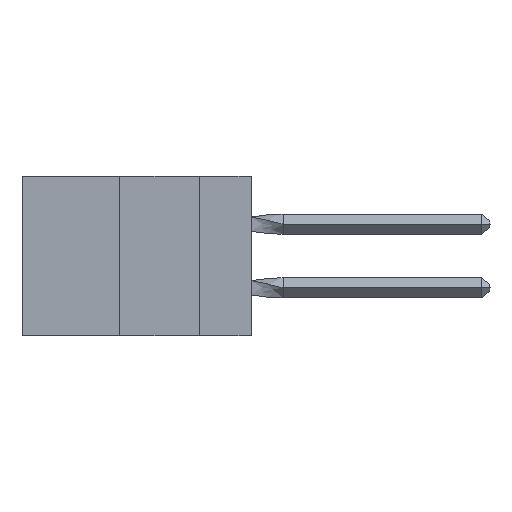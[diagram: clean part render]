
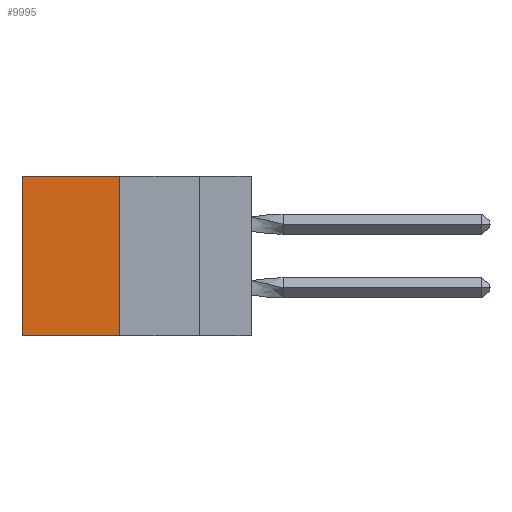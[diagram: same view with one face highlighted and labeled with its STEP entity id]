
A CAD part, left-side view. The second image highlights one B-rep face of the part: STEP entity #9995.
In plain terms, the highlighted planar face has unit normal (-1, 0, 0).
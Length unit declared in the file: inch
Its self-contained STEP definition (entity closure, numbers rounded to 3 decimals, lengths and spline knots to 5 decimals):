
#603 = LINE ( 'NONE', #24592, #18379 ) ;
#637 = CARTESIAN_POINT ( 'NONE',  ( 0.305, 0.413, 0. ) ) ;
#692 = FACE_OUTER_BOUND ( 'NONE', #27209, .T. ) ;
#999 = LINE ( 'NONE', #6734, #24939 ) ;
#2280 = DIRECTION ( 'NONE',  ( 0., 0., -1. ) ) ;
#2689 = VERTEX_POINT ( 'NONE', #19677 ) ;
#2735 = VECTOR ( 'NONE', #25598, 39.37008 ) ;
#3597 = PLANE ( 'NONE',  #12954 ) ;
#4885 = VERTEX_POINT ( 'NONE', #9033 ) ;
#5884 = EDGE_CURVE ( 'NONE', #26504, #4885, #999, .T. ) ;
#6734 = CARTESIAN_POINT ( 'NONE',  ( 0.305, 0.413, -0.5 ) ) ;
#8428 = ORIENTED_EDGE ( 'NONE', *, *, #5884, .F. ) ;
#8508 = CARTESIAN_POINT ( 'NONE',  ( 0.305, 0.72, -0.5 ) ) ;
#9033 = CARTESIAN_POINT ( 'NONE',  ( 0.305, 0.72, -0.5 ) ) ;
#9249 = DIRECTION ( 'NONE',  ( 0., 1., 0. ) ) ;
#9995 = ADVANCED_FACE ( 'NONE', ( #692 ), #3597, .F. ) ;
#10556 = CARTESIAN_POINT ( 'NONE',  ( 0.305, 0.413, -0.5 ) ) ;
#10944 = DIRECTION ( 'NONE',  ( 0., 0., -1. ) ) ;
#12571 = VECTOR ( 'NONE', #13530, 39.37008 ) ;
#12954 = AXIS2_PLACEMENT_3D ( 'NONE', #25683, #28383, #10944 ) ;
#13207 = CARTESIAN_POINT ( 'NONE',  ( 0.305, 0.413, 0. ) ) ;
#13530 = DIRECTION ( 'NONE',  ( 0., 1., 0. ) ) ;
#16539 = EDGE_CURVE ( 'NONE', #2689, #4885, #28957, .T. ) ;
#18379 = VECTOR ( 'NONE', #2280, 39.37008 ) ;
#18786 = EDGE_CURVE ( 'NONE', #24876, #26504, #603, .T. ) ;
#19497 = ORIENTED_EDGE ( 'NONE', *, *, #28671, .T. ) ;
#19677 = CARTESIAN_POINT ( 'NONE',  ( 0.305, 0.72, 0. ) ) ;
#24592 = CARTESIAN_POINT ( 'NONE',  ( 0.305, 0.413, -0.5 ) ) ;
#24876 = VERTEX_POINT ( 'NONE', #637 ) ;
#24939 = VECTOR ( 'NONE', #9249, 39.37008 ) ;
#25598 = DIRECTION ( 'NONE',  ( 0., 0., -1. ) ) ;
#25683 = CARTESIAN_POINT ( 'NONE',  ( 0.305, 0.413, -0.5 ) ) ;
#26504 = VERTEX_POINT ( 'NONE', #10556 ) ;
#27173 = ORIENTED_EDGE ( 'NONE', *, *, #18786, .F. ) ;
#27209 = EDGE_LOOP ( 'NONE', ( #30562, #8428, #27173, #19497 ) ) ;
#28383 = DIRECTION ( 'NONE',  ( 1., 0., 0. ) ) ;
#28671 = EDGE_CURVE ( 'NONE', #24876, #2689, #29940, .T. ) ;
#28957 = LINE ( 'NONE', #8508, #2735 ) ;
#29940 = LINE ( 'NONE', #13207, #12571 ) ;
#30562 = ORIENTED_EDGE ( 'NONE', *, *, #16539, .T. ) ;
